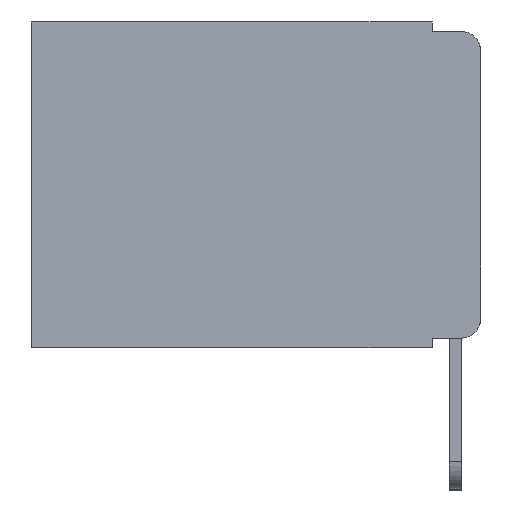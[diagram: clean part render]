
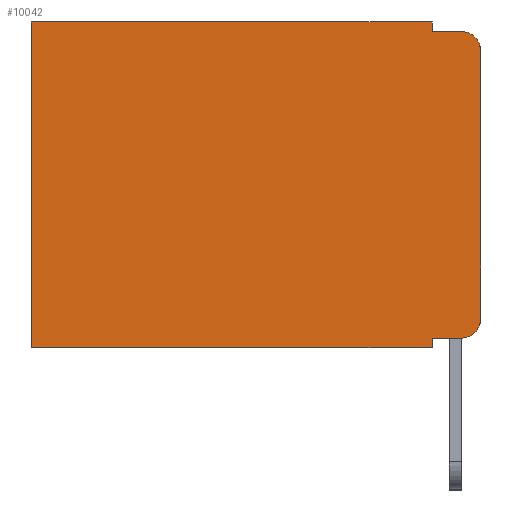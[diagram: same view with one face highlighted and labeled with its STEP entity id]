
A CAD part, left-side view. The second image highlights one B-rep face of the part: STEP entity #10042.
In plain terms, the highlighted planar face has unit normal (-1, 0, 0).
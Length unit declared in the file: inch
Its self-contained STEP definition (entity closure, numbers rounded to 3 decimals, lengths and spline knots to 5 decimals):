
#279 = EDGE_CURVE ( 'NONE', #898, #3120, #15139, .T. ) ;
#649 = LINE ( 'NONE', #10544, #15242 ) ;
#725 = CARTESIAN_POINT ( 'NONE',  ( 0.298, 0.02, -0.333 ) ) ;
#740 = PLANE ( 'NONE',  #5733 ) ;
#898 = VERTEX_POINT ( 'NONE', #13985 ) ;
#1139 = LINE ( 'NONE', #9290, #6581 ) ;
#1146 = ORIENTED_EDGE ( 'NONE', *, *, #8274, .T. ) ;
#1204 = VERTEX_POINT ( 'NONE', #6746 ) ;
#1347 = CARTESIAN_POINT ( 'NONE',  ( 0.298, 0.02, -0.313 ) ) ;
#1837 = CARTESIAN_POINT ( 'NONE',  ( 0.298, 0.051, -0.343 ) ) ;
#1866 = VERTEX_POINT ( 'NONE', #16147 ) ;
#1882 = EDGE_CURVE ( 'NONE', #15312, #4007, #5759, .T. ) ;
#1910 = EDGE_CURVE ( 'NONE', #1204, #3120, #15288, .T. ) ;
#2437 = ORIENTED_EDGE ( 'NONE', *, *, #1910, .T. ) ;
#2801 = AXIS2_PLACEMENT_3D ( 'NONE', #10140, #11177, #3905 ) ;
#3120 = VERTEX_POINT ( 'NONE', #14720 ) ;
#3186 = EDGE_CURVE ( 'NONE', #13326, #15312, #15645, .T. ) ;
#3367 = EDGE_CURVE ( 'NONE', #1204, #4007, #649, .T. ) ;
#3426 = ORIENTED_EDGE ( 'NONE', *, *, #12835, .F. ) ;
#3486 = ORIENTED_EDGE ( 'NONE', *, *, #279, .F. ) ;
#3855 = LINE ( 'NONE', #13884, #16124 ) ;
#3905 = DIRECTION ( 'NONE',  ( 0., 0., -1. ) ) ;
#4007 = VERTEX_POINT ( 'NONE', #12947 ) ;
#4184 = DIRECTION ( 'NONE',  ( 0., 1., 0. ) ) ;
#4358 = VERTEX_POINT ( 'NONE', #7363 ) ;
#4392 = DIRECTION ( 'NONE',  ( 0., 0., -1. ) ) ;
#4718 = EDGE_LOOP ( 'NONE', ( #8984, #2437, #3486, #3426, #1146, #7592, #15728, #7201, #6059, #11143 ) ) ;
#4732 = DIRECTION ( 'NONE',  ( 0., 0., -1. ) ) ;
#4985 = CARTESIAN_POINT ( 'NONE',  ( 0.298, 0.051, 0. ) ) ;
#5038 = VECTOR ( 'NONE', #4732, 39.37008 ) ;
#5485 = DIRECTION ( 'NONE',  ( 0., -1., 0. ) ) ;
#5733 = AXIS2_PLACEMENT_3D ( 'NONE', #9390, #10567, #4392 ) ;
#5759 = CIRCLE ( 'NONE', #8610, 0.02 ) ;
#6059 = ORIENTED_EDGE ( 'NONE', *, *, #3186, .T. ) ;
#6079 = VECTOR ( 'NONE', #11171, 39.37008 ) ;
#6338 = DIRECTION ( 'NONE',  ( 0., 0., -1. ) ) ;
#6581 = VECTOR ( 'NONE', #7904, 39.37008 ) ;
#6622 = CARTESIAN_POINT ( 'NONE',  ( 0.298, 0.051, 0. ) ) ;
#6746 = CARTESIAN_POINT ( 'NONE',  ( 0.298, 0., -0.03 ) ) ;
#7201 = ORIENTED_EDGE ( 'NONE', *, *, #10121, .F. ) ;
#7363 = CARTESIAN_POINT ( 'NONE',  ( 0.298, 0.473, 0. ) ) ;
#7592 = ORIENTED_EDGE ( 'NONE', *, *, #8094, .T. ) ;
#7671 = LINE ( 'NONE', #15804, #13944 ) ;
#7904 = DIRECTION ( 'NONE',  ( 0., 1., 0. ) ) ;
#8094 = EDGE_CURVE ( 'NONE', #4358, #1866, #11657, .T. ) ;
#8235 = EDGE_CURVE ( 'NONE', #14867, #1866, #3855, .T. ) ;
#8274 = EDGE_CURVE ( 'NONE', #8302, #4358, #1139, .T. ) ;
#8302 = VERTEX_POINT ( 'NONE', #6622 ) ;
#8610 = AXIS2_PLACEMENT_3D ( 'NONE', #1347, #8848, #6338 ) ;
#8848 = DIRECTION ( 'NONE',  ( -1., 0., 0. ) ) ;
#8984 = ORIENTED_EDGE ( 'NONE', *, *, #3367, .F. ) ;
#9054 = CARTESIAN_POINT ( 'NONE',  ( 0.298, 0.051, -0.333 ) ) ;
#9290 = CARTESIAN_POINT ( 'NONE',  ( 0.298, 0., 0. ) ) ;
#9390 = CARTESIAN_POINT ( 'NONE',  ( 0.298, 0., 0. ) ) ;
#9945 = LINE ( 'NONE', #4985, #6079 ) ;
#10042 = ADVANCED_FACE ( 'NONE', ( #14123 ), #740, .F. ) ;
#10121 = EDGE_CURVE ( 'NONE', #13326, #14867, #7671, .T. ) ;
#10140 = CARTESIAN_POINT ( 'NONE',  ( 0.298, 0.02, -0.03 ) ) ;
#10544 = CARTESIAN_POINT ( 'NONE',  ( 0.298, 0., 0. ) ) ;
#10567 = DIRECTION ( 'NONE',  ( 1., 0., 0. ) ) ;
#11143 = ORIENTED_EDGE ( 'NONE', *, *, #1882, .T. ) ;
#11171 = DIRECTION ( 'NONE',  ( 0., 0., -1. ) ) ;
#11177 = DIRECTION ( 'NONE',  ( -1., 0., 0. ) ) ;
#11657 = LINE ( 'NONE', #14590, #5038 ) ;
#11839 = VECTOR ( 'NONE', #5485, 39.37008 ) ;
#12835 = EDGE_CURVE ( 'NONE', #8302, #898, #9945, .T. ) ;
#12947 = CARTESIAN_POINT ( 'NONE',  ( 0.298, 0., -0.313 ) ) ;
#13326 = VERTEX_POINT ( 'NONE', #15964 ) ;
#13411 = DIRECTION ( 'NONE',  ( 0., 0., -1. ) ) ;
#13884 = CARTESIAN_POINT ( 'NONE',  ( 0.298, 0., -0.343 ) ) ;
#13944 = VECTOR ( 'NONE', #13411, 39.37008 ) ;
#13985 = CARTESIAN_POINT ( 'NONE',  ( 0.298, 0.051, -0.01 ) ) ;
#14123 = FACE_OUTER_BOUND ( 'NONE', #4718, .T. ) ;
#14135 = CARTESIAN_POINT ( 'NONE',  ( 0.298, 0.051, -0.01 ) ) ;
#14570 = DIRECTION ( 'NONE',  ( 0., 0., -1. ) ) ;
#14590 = CARTESIAN_POINT ( 'NONE',  ( 0.298, 0.473, 0. ) ) ;
#14720 = CARTESIAN_POINT ( 'NONE',  ( 0.298, 0.02, -0.01 ) ) ;
#14867 = VERTEX_POINT ( 'NONE', #1837 ) ;
#15139 = LINE ( 'NONE', #14135, #11839 ) ;
#15242 = VECTOR ( 'NONE', #14570, 39.37008 ) ;
#15255 = DIRECTION ( 'NONE',  ( 0., -1., 0. ) ) ;
#15288 = CIRCLE ( 'NONE', #2801, 0.02 ) ;
#15312 = VERTEX_POINT ( 'NONE', #725 ) ;
#15645 = LINE ( 'NONE', #9054, #16020 ) ;
#15728 = ORIENTED_EDGE ( 'NONE', *, *, #8235, .F. ) ;
#15804 = CARTESIAN_POINT ( 'NONE',  ( 0.298, 0.051, 0. ) ) ;
#15964 = CARTESIAN_POINT ( 'NONE',  ( 0.298, 0.051, -0.333 ) ) ;
#16020 = VECTOR ( 'NONE', #15255, 39.37008 ) ;
#16124 = VECTOR ( 'NONE', #4184, 39.37008 ) ;
#16147 = CARTESIAN_POINT ( 'NONE',  ( 0.298, 0.473, -0.343 ) ) ;
